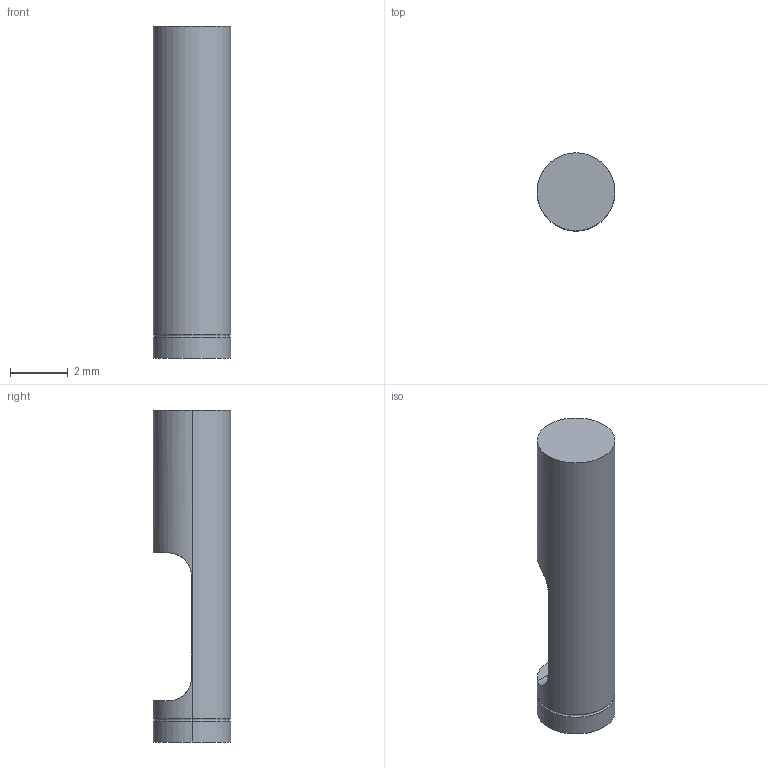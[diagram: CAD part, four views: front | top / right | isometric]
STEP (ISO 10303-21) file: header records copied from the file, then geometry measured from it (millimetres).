
FILE_DESCRIPTION (( 'STEP AP214' ), '1' );
FILE_NAME ('User Library-M4A1 - Bolt Carrier - Assembly_M4A1 - Bolt - Ejector1.STEP', '2013-05-23T12:52:58', ( 'Asher' ), ( '' ), 'SwSTEP 2.0', 'SolidWorks 2013', '' );
FILE_SCHEMA (( 'AUTOMOTIVE_DESIGN' ));
Length unit declared in the file: millimetre
Products named in the file (1): User Library-M4A1 - Bolt Carrier - Assembly_M4A1 - Bolt - Ejector1
Bounding box: 2.7 x 2.7 x 11.51 mm (x, y, z)
Volume: 52.1 mm3; surface area: 106 mm2
Topology: 1 solids, 1 shells, 13 faces, 26 edges, 16 vertices
Faces by surface type: cylinder 6, plane 5, bspline 2
Entity records: 424 total; most frequent: CARTESIAN_POINT 122, DIRECTION 58, ORIENTED_EDGE 52, EDGE_CURVE 26, AXIS2_PLACEMENT_3D 24, VERTEX_POINT 16, EDGE_LOOP 14, FACE_OUTER_BOUND 13
